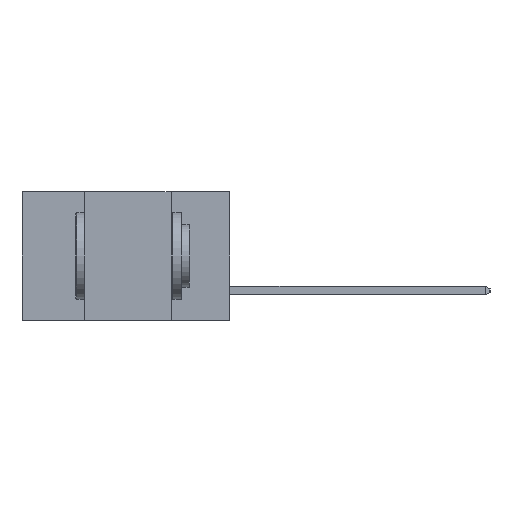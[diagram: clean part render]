
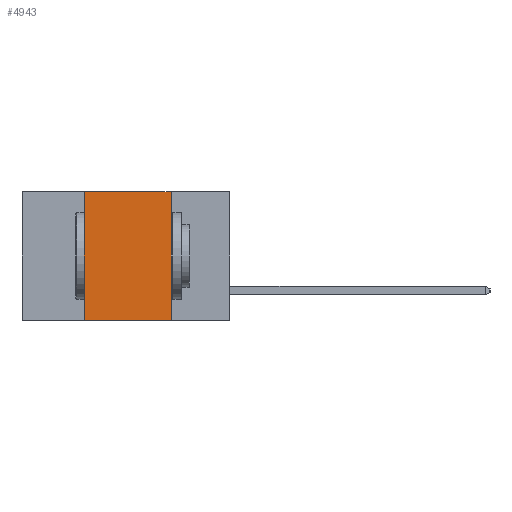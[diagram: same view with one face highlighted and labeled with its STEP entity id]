
A CAD part, left-side view. The second image highlights one B-rep face of the part: STEP entity #4943.
In plain terms, the highlighted planar face has unit normal (-1, 0, 0).
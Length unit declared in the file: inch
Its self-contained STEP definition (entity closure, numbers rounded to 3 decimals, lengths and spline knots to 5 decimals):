
#93 = DIRECTION ( 'NONE',  ( 0., 0., 1. ) ) ;
#160 = DIRECTION ( 'NONE',  ( 0., -1., 0. ) ) ;
#194 = CARTESIAN_POINT ( 'NONE',  ( 0., 0.17, -0.37 ) ) ;
#1829 = EDGE_CURVE ( 'NONE', #23611, #6561, #28656, .T. ) ;
#2559 = CARTESIAN_POINT ( 'NONE',  ( 0., 0.6, -0.37 ) ) ;
#2858 = CARTESIAN_POINT ( 'NONE',  ( 0., 0.42, 0. ) ) ;
#4520 = EDGE_CURVE ( 'NONE', #20510, #28613, #26237, .T. ) ;
#4943 = ADVANCED_FACE ( 'NONE', ( #11509 ), #7325, .F. ) ;
#5185 = CARTESIAN_POINT ( 'NONE',  ( 0., 0.6, 0. ) ) ;
#5332 = DIRECTION ( 'NONE',  ( 1., 0., 0. ) ) ;
#6561 = VERTEX_POINT ( 'NONE', #194 ) ;
#7325 = PLANE ( 'NONE',  #25769 ) ;
#7936 = CARTESIAN_POINT ( 'NONE',  ( 0., 0.6, 0. ) ) ;
#9518 = VECTOR ( 'NONE', #24671, 39.37008 ) ;
#11509 = FACE_OUTER_BOUND ( 'NONE', #27643, .T. ) ;
#11567 = CARTESIAN_POINT ( 'NONE',  ( 0., 0.42, 0. ) ) ;
#12335 = LINE ( 'NONE', #2559, #22930 ) ;
#13432 = LINE ( 'NONE', #7936, #19094 ) ;
#14440 = CARTESIAN_POINT ( 'NONE',  ( 0., 0.42, -0.37 ) ) ;
#17558 = DIRECTION ( 'NONE',  ( 0., -1., 0. ) ) ;
#17626 = CARTESIAN_POINT ( 'NONE',  ( 0., 0.17, 0. ) ) ;
#17671 = ORIENTED_EDGE ( 'NONE', *, *, #1829, .F. ) ;
#17702 = ORIENTED_EDGE ( 'NONE', *, *, #30745, .F. ) ;
#17974 = DIRECTION ( 'NONE',  ( 0., 0., -1. ) ) ;
#19094 = VECTOR ( 'NONE', #17558, 39.37008 ) ;
#20349 = ORIENTED_EDGE ( 'NONE', *, *, #26982, .T. ) ;
#20510 = VERTEX_POINT ( 'NONE', #14440 ) ;
#21490 = ORIENTED_EDGE ( 'NONE', *, *, #4520, .F. ) ;
#22930 = VECTOR ( 'NONE', #160, 39.37008 ) ;
#23611 = VERTEX_POINT ( 'NONE', #17626 ) ;
#24671 = DIRECTION ( 'NONE',  ( 0., 0., -1. ) ) ;
#24777 = VECTOR ( 'NONE', #93, 39.37008 ) ;
#24983 = CARTESIAN_POINT ( 'NONE',  ( 0., 0.17, 0. ) ) ;
#25769 = AXIS2_PLACEMENT_3D ( 'NONE', #5185, #5332, #17974 ) ;
#26237 = LINE ( 'NONE', #2858, #24777 ) ;
#26982 = EDGE_CURVE ( 'NONE', #20510, #6561, #12335, .T. ) ;
#27643 = EDGE_LOOP ( 'NONE', ( #17671, #17702, #21490, #20349 ) ) ;
#28613 = VERTEX_POINT ( 'NONE', #11567 ) ;
#28656 = LINE ( 'NONE', #24983, #9518 ) ;
#30745 = EDGE_CURVE ( 'NONE', #28613, #23611, #13432, .T. ) ;
